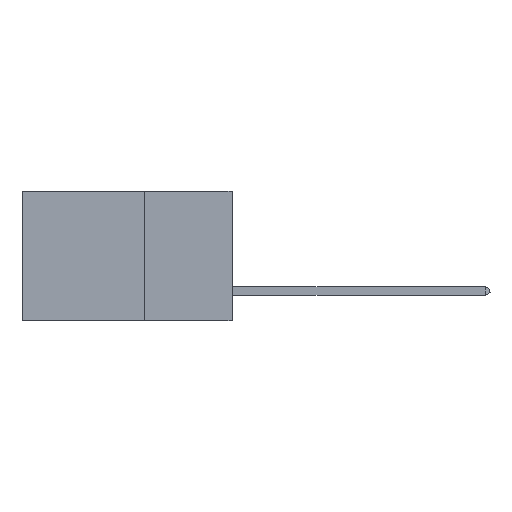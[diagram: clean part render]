
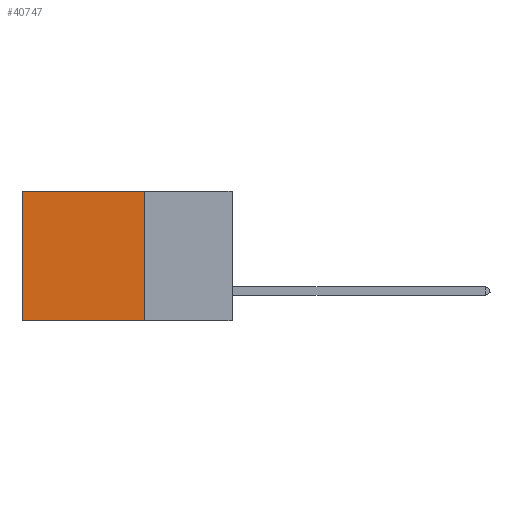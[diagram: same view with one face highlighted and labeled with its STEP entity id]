
A CAD part, left-side view. The second image highlights one B-rep face of the part: STEP entity #40747.
In plain terms, the highlighted planar face has unit normal (-1, 0, 0).
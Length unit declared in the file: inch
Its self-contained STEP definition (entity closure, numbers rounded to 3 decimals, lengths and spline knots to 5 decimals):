
#1558 = DIRECTION ( 'NONE',  ( 0., 1., 0. ) ) ;
#1581 = CARTESIAN_POINT ( 'NONE',  ( 0.2875, 0.25, 0. ) ) ;
#2684 = EDGE_CURVE ( 'NONE', #7029, #10461, #33512, .T. ) ;
#3180 = CARTESIAN_POINT ( 'NONE',  ( 0.2875, 0.25, -0.37 ) ) ;
#3236 = LINE ( 'NONE', #12865, #17419 ) ;
#7029 = VERTEX_POINT ( 'NONE', #42596 ) ;
#7755 = VECTOR ( 'NONE', #30242, 39.37008 ) ;
#8571 = DIRECTION ( 'NONE',  ( 1., 0., 0. ) ) ;
#9769 = DIRECTION ( 'NONE',  ( 0., 0., -1. ) ) ;
#10461 = VERTEX_POINT ( 'NONE', #36568 ) ;
#11830 = FACE_OUTER_BOUND ( 'NONE', #22730, .T. ) ;
#12573 = VECTOR ( 'NONE', #1558, 39.37008 ) ;
#12865 = CARTESIAN_POINT ( 'NONE',  ( 0.2875, 0.6, 0. ) ) ;
#13579 = VERTEX_POINT ( 'NONE', #3180 ) ;
#17419 = VECTOR ( 'NONE', #26153, 39.37008 ) ;
#20473 = LINE ( 'NONE', #40127, #25824 ) ;
#22663 = EDGE_CURVE ( 'NONE', #13579, #31177, #25339, .T. ) ;
#22730 = EDGE_LOOP ( 'NONE', ( #30438, #30935, #40909, #31528 ) ) ;
#23408 = EDGE_CURVE ( 'NONE', #7029, #13579, #20473, .T. ) ;
#23615 = CARTESIAN_POINT ( 'NONE',  ( 0.2875, 0.6, -0.37 ) ) ;
#24422 = AXIS2_PLACEMENT_3D ( 'NONE', #1581, #8571, #31490 ) ;
#25339 = LINE ( 'NONE', #31470, #12573 ) ;
#25824 = VECTOR ( 'NONE', #9769, 39.37008 ) ;
#26153 = DIRECTION ( 'NONE',  ( 0., 0., -1. ) ) ;
#30242 = DIRECTION ( 'NONE',  ( 0., 1., 0. ) ) ;
#30438 = ORIENTED_EDGE ( 'NONE', *, *, #40003, .T. ) ;
#30935 = ORIENTED_EDGE ( 'NONE', *, *, #22663, .F. ) ;
#31177 = VERTEX_POINT ( 'NONE', #23615 ) ;
#31470 = CARTESIAN_POINT ( 'NONE',  ( 0.2875, 0.25, -0.37 ) ) ;
#31490 = DIRECTION ( 'NONE',  ( 0., 0., -1. ) ) ;
#31528 = ORIENTED_EDGE ( 'NONE', *, *, #2684, .T. ) ;
#32349 = PLANE ( 'NONE',  #24422 ) ;
#33293 = CARTESIAN_POINT ( 'NONE',  ( 0.2875, 0.25, 0. ) ) ;
#33512 = LINE ( 'NONE', #33293, #7755 ) ;
#36568 = CARTESIAN_POINT ( 'NONE',  ( 0.2875, 0.6, 0. ) ) ;
#40003 = EDGE_CURVE ( 'NONE', #10461, #31177, #3236, .T. ) ;
#40127 = CARTESIAN_POINT ( 'NONE',  ( 0.2875, 0.25, 0. ) ) ;
#40747 = ADVANCED_FACE ( 'NONE', ( #11830 ), #32349, .F. ) ;
#40909 = ORIENTED_EDGE ( 'NONE', *, *, #23408, .F. ) ;
#42596 = CARTESIAN_POINT ( 'NONE',  ( 0.2875, 0.25, 0. ) ) ;
